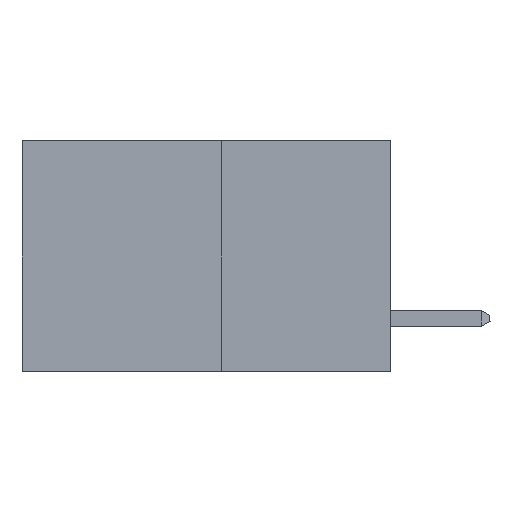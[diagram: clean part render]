
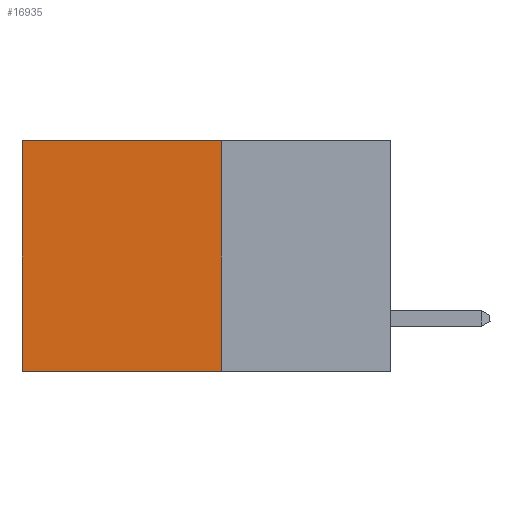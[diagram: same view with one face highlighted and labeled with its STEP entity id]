
A CAD part, left-side view. The second image highlights one B-rep face of the part: STEP entity #16935.
In plain terms, the highlighted planar face has unit normal (-1, 0, 0).
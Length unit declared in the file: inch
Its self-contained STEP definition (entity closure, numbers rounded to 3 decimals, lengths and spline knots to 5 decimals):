
#674 = CARTESIAN_POINT ( 'NONE',  ( 0.277, 0.27, -0.37 ) ) ;
#1067 = CARTESIAN_POINT ( 'NONE',  ( 0.277, 0.59, 0. ) ) ;
#3938 = VECTOR ( 'NONE', #9412, 39.37008 ) ;
#4097 = EDGE_CURVE ( 'NONE', #19447, #17014, #14057, .T. ) ;
#4358 = LINE ( 'NONE', #7789, #4991 ) ;
#4991 = VECTOR ( 'NONE', #11802, 39.37008 ) ;
#6916 = PLANE ( 'NONE',  #8600 ) ;
#7489 = VECTOR ( 'NONE', #15169, 39.37008 ) ;
#7789 = CARTESIAN_POINT ( 'NONE',  ( 0.277, 0.27, 0. ) ) ;
#8600 = AXIS2_PLACEMENT_3D ( 'NONE', #674, #20971, #9001 ) ;
#9001 = DIRECTION ( 'NONE',  ( 0., 0., -1. ) ) ;
#9284 = CARTESIAN_POINT ( 'NONE',  ( 0.277, 0.27, -0.37 ) ) ;
#9412 = DIRECTION ( 'NONE',  ( 0., 1., 0. ) ) ;
#10479 = EDGE_CURVE ( 'NONE', #14691, #17014, #11553, .T. ) ;
#10660 = ORIENTED_EDGE ( 'NONE', *, *, #4097, .F. ) ;
#11553 = LINE ( 'NONE', #13172, #7489 ) ;
#11802 = DIRECTION ( 'NONE',  ( 0., 1., 0. ) ) ;
#12057 = CARTESIAN_POINT ( 'NONE',  ( 0.277, 0.27, -0.37 ) ) ;
#12411 = CARTESIAN_POINT ( 'NONE',  ( 0.277, 0.27, 0. ) ) ;
#13172 = CARTESIAN_POINT ( 'NONE',  ( 0.277, 0.59, -0.37 ) ) ;
#14057 = LINE ( 'NONE', #9284, #3938 ) ;
#14066 = DIRECTION ( 'NONE',  ( 0., 0., -1. ) ) ;
#14484 = CARTESIAN_POINT ( 'NONE',  ( 0.277, 0.27, -0.37 ) ) ;
#14691 = VERTEX_POINT ( 'NONE', #1067 ) ;
#15169 = DIRECTION ( 'NONE',  ( 0., 0., -1. ) ) ;
#16074 = FACE_OUTER_BOUND ( 'NONE', #19187, .T. ) ;
#16935 = ADVANCED_FACE ( 'NONE', ( #16074 ), #6916, .F. ) ;
#16945 = VECTOR ( 'NONE', #14066, 39.37008 ) ;
#17014 = VERTEX_POINT ( 'NONE', #17142 ) ;
#17142 = CARTESIAN_POINT ( 'NONE',  ( 0.277, 0.59, -0.37 ) ) ;
#17970 = EDGE_CURVE ( 'NONE', #21327, #19447, #23505, .T. ) ;
#18513 = ORIENTED_EDGE ( 'NONE', *, *, #21073, .T. ) ;
#19187 = EDGE_LOOP ( 'NONE', ( #25764, #10660, #24142, #18513 ) ) ;
#19447 = VERTEX_POINT ( 'NONE', #14484 ) ;
#20971 = DIRECTION ( 'NONE',  ( 1., 0., 0. ) ) ;
#21073 = EDGE_CURVE ( 'NONE', #21327, #14691, #4358, .T. ) ;
#21327 = VERTEX_POINT ( 'NONE', #12411 ) ;
#23505 = LINE ( 'NONE', #12057, #16945 ) ;
#24142 = ORIENTED_EDGE ( 'NONE', *, *, #17970, .F. ) ;
#25764 = ORIENTED_EDGE ( 'NONE', *, *, #10479, .T. ) ;
